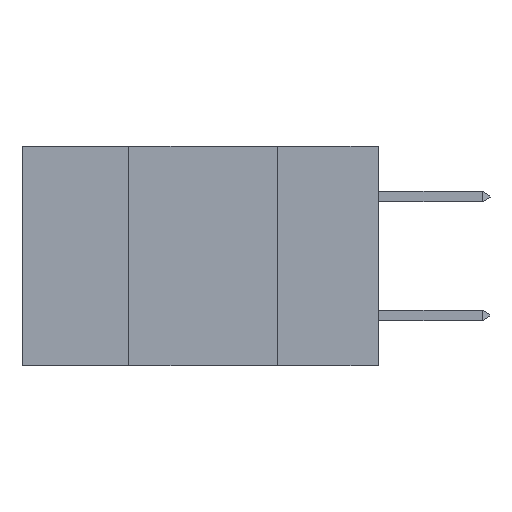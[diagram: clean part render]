
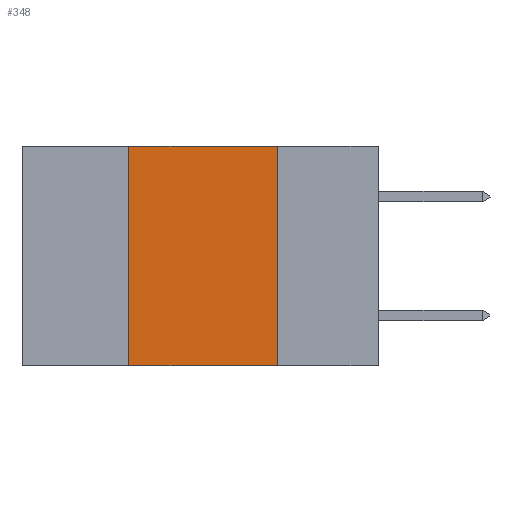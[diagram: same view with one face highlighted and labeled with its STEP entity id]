
A CAD part, left-side view. The second image highlights one B-rep face of the part: STEP entity #348.
In plain terms, the highlighted planar face has unit normal (-1, 0, 0).
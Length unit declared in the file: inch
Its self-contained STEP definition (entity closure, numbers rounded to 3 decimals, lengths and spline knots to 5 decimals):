
#100 = AXIS2_PLACEMENT_3D ( 'NONE', #6243, #7895, #4325 ) ;
#140 = ORIENTED_EDGE ( 'NONE', *, *, #6451, .T. ) ;
#257 = FACE_OUTER_BOUND ( 'NONE', #5071, .T. ) ;
#348 = ADVANCED_FACE ( 'NONE', ( #257 ), #8795, .F. ) ;
#448 = VECTOR ( 'NONE', #1480, 39.37008 ) ;
#472 = LINE ( 'NONE', #8233, #10888 ) ;
#697 = CARTESIAN_POINT ( 'NONE',  ( 0., 0.17, -0.37 ) ) ;
#1048 = LINE ( 'NONE', #10037, #6628 ) ;
#1434 = CARTESIAN_POINT ( 'NONE',  ( 0., 0.17, 0. ) ) ;
#1480 = DIRECTION ( 'NONE',  ( 0., -1., 0. ) ) ;
#2912 = LINE ( 'NONE', #5881, #448 ) ;
#3223 = EDGE_CURVE ( 'NONE', #11303, #4930, #1048, .T. ) ;
#4325 = DIRECTION ( 'NONE',  ( 0., 0., -1. ) ) ;
#4536 = CARTESIAN_POINT ( 'NONE',  ( 0., 0.42, 0. ) ) ;
#4804 = EDGE_CURVE ( 'NONE', #10003, #11303, #7018, .T. ) ;
#4910 = CARTESIAN_POINT ( 'NONE',  ( 0., 0.42, -0.37 ) ) ;
#4930 = VERTEX_POINT ( 'NONE', #697 ) ;
#5071 = EDGE_LOOP ( 'NONE', ( #10784, #7408, #9300, #140 ) ) ;
#5881 = CARTESIAN_POINT ( 'NONE',  ( 0., 0.6, -0.37 ) ) ;
#6243 = CARTESIAN_POINT ( 'NONE',  ( 0., 0.6, 0. ) ) ;
#6451 = EDGE_CURVE ( 'NONE', #8441, #4930, #2912, .T. ) ;
#6535 = DIRECTION ( 'NONE',  ( 0., -1., 0. ) ) ;
#6628 = VECTOR ( 'NONE', #10111, 39.37008 ) ;
#7018 = LINE ( 'NONE', #7343, #10222 ) ;
#7343 = CARTESIAN_POINT ( 'NONE',  ( 0., 0.6, 0. ) ) ;
#7408 = ORIENTED_EDGE ( 'NONE', *, *, #4804, .F. ) ;
#7895 = DIRECTION ( 'NONE',  ( 1., 0., 0. ) ) ;
#8115 = EDGE_CURVE ( 'NONE', #8441, #10003, #472, .T. ) ;
#8233 = CARTESIAN_POINT ( 'NONE',  ( 0., 0.42, 0. ) ) ;
#8441 = VERTEX_POINT ( 'NONE', #4910 ) ;
#8795 = PLANE ( 'NONE',  #100 ) ;
#9011 = DIRECTION ( 'NONE',  ( 0., 0., 1. ) ) ;
#9300 = ORIENTED_EDGE ( 'NONE', *, *, #8115, .F. ) ;
#10003 = VERTEX_POINT ( 'NONE', #4536 ) ;
#10037 = CARTESIAN_POINT ( 'NONE',  ( 0., 0.17, 0. ) ) ;
#10111 = DIRECTION ( 'NONE',  ( 0., 0., -1. ) ) ;
#10222 = VECTOR ( 'NONE', #6535, 39.37008 ) ;
#10784 = ORIENTED_EDGE ( 'NONE', *, *, #3223, .F. ) ;
#10888 = VECTOR ( 'NONE', #9011, 39.37008 ) ;
#11303 = VERTEX_POINT ( 'NONE', #1434 ) ;
